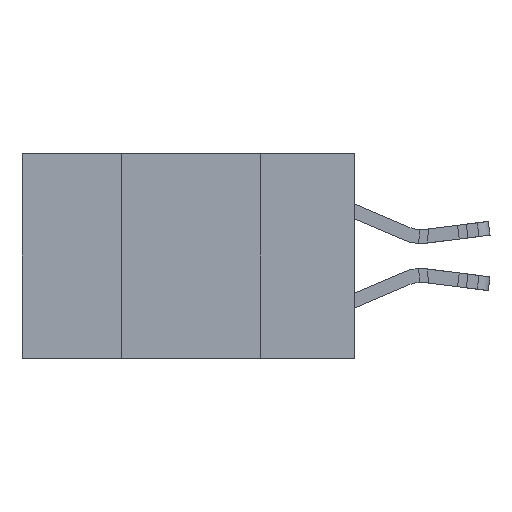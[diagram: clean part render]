
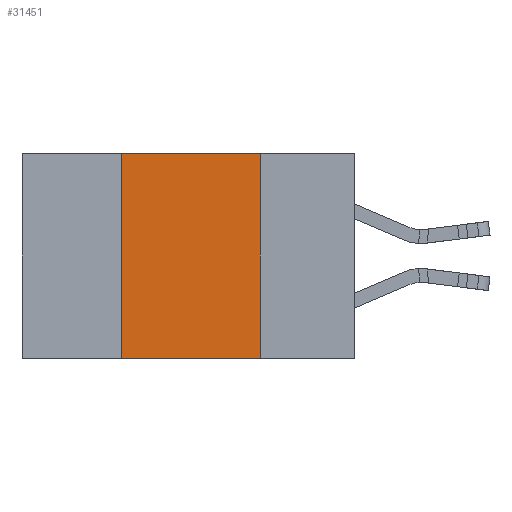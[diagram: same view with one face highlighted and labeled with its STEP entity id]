
A CAD part, left-side view. The second image highlights one B-rep face of the part: STEP entity #31451.
In plain terms, the highlighted planar face has unit normal (-1, 0, 0).
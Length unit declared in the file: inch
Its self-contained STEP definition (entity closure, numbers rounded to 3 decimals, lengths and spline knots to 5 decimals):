
#110 = ORIENTED_EDGE ( 'NONE', *, *, #32390, .F. ) ;
#1127 = CARTESIAN_POINT ( 'NONE',  ( 0., 0.6, -0.37 ) ) ;
#1227 = DIRECTION ( 'NONE',  ( 0., -1., 0. ) ) ;
#1748 = DIRECTION ( 'NONE',  ( 1., 0., 0. ) ) ;
#2893 = VECTOR ( 'NONE', #8288, 39.37008 ) ;
#3683 = ORIENTED_EDGE ( 'NONE', *, *, #29731, .F. ) ;
#5533 = VERTEX_POINT ( 'NONE', #30490 ) ;
#5741 = CARTESIAN_POINT ( 'NONE',  ( 0., 0.42, 0. ) ) ;
#6132 = LINE ( 'NONE', #15810, #25674 ) ;
#6904 = VERTEX_POINT ( 'NONE', #27195 ) ;
#6967 = FACE_OUTER_BOUND ( 'NONE', #9945, .T. ) ;
#8180 = DIRECTION ( 'NONE',  ( 0., 0., -1. ) ) ;
#8288 = DIRECTION ( 'NONE',  ( 0., 0., 1. ) ) ;
#9263 = ORIENTED_EDGE ( 'NONE', *, *, #29680, .T. ) ;
#9945 = EDGE_LOOP ( 'NONE', ( #13232, #3683, #110, #9263 ) ) ;
#10469 = LINE ( 'NONE', #5741, #2893 ) ;
#11255 = DIRECTION ( 'NONE',  ( 0., -1., 0. ) ) ;
#12251 = EDGE_CURVE ( 'NONE', #6904, #19025, #6132, .T. ) ;
#13085 = LINE ( 'NONE', #1127, #26667 ) ;
#13232 = ORIENTED_EDGE ( 'NONE', *, *, #12251, .F. ) ;
#15250 = VERTEX_POINT ( 'NONE', #15684 ) ;
#15684 = CARTESIAN_POINT ( 'NONE',  ( 0., 0.42, -0.37 ) ) ;
#15810 = CARTESIAN_POINT ( 'NONE',  ( 0., 0.17, 0. ) ) ;
#17081 = PLANE ( 'NONE',  #31433 ) ;
#19025 = VERTEX_POINT ( 'NONE', #22527 ) ;
#19100 = LINE ( 'NONE', #19111, #25050 ) ;
#19111 = CARTESIAN_POINT ( 'NONE',  ( 0., 0.6, 0. ) ) ;
#19628 = DIRECTION ( 'NONE',  ( 0., 0., -1. ) ) ;
#22527 = CARTESIAN_POINT ( 'NONE',  ( 0., 0.17, -0.37 ) ) ;
#25050 = VECTOR ( 'NONE', #1227, 39.37008 ) ;
#25674 = VECTOR ( 'NONE', #8180, 39.37008 ) ;
#26667 = VECTOR ( 'NONE', #11255, 39.37008 ) ;
#27195 = CARTESIAN_POINT ( 'NONE',  ( 0., 0.17, 0. ) ) ;
#29680 = EDGE_CURVE ( 'NONE', #15250, #19025, #13085, .T. ) ;
#29731 = EDGE_CURVE ( 'NONE', #5533, #6904, #19100, .T. ) ;
#30490 = CARTESIAN_POINT ( 'NONE',  ( 0., 0.42, 0. ) ) ;
#31433 = AXIS2_PLACEMENT_3D ( 'NONE', #32251, #1748, #19628 ) ;
#31451 = ADVANCED_FACE ( 'NONE', ( #6967 ), #17081, .F. ) ;
#32251 = CARTESIAN_POINT ( 'NONE',  ( 0., 0.6, 0. ) ) ;
#32390 = EDGE_CURVE ( 'NONE', #15250, #5533, #10469, .T. ) ;
